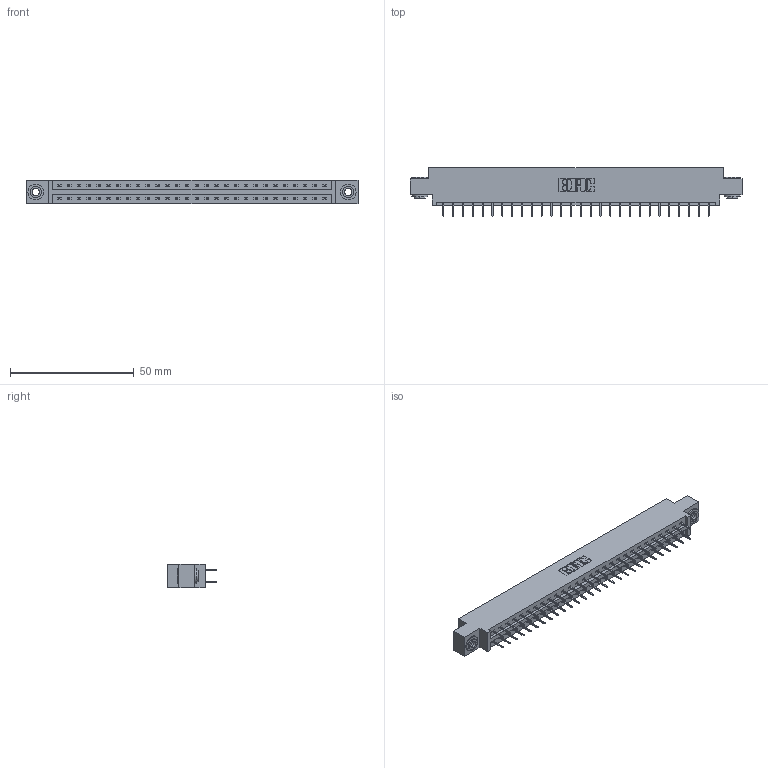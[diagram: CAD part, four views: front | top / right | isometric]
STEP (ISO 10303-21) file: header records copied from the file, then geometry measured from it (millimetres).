
FILE_DESCRIPTION (( 'STEP AP203' ), '1' );
FILE_NAME ('387-056-524-803.STEP', '2019-10-19T06:42:10', ( '' ), ( '' ), 'SwSTEP 2.0', 'SolidWorks 2016', '' );
FILE_SCHEMA (( 'CONFIG_CONTROL_DESIGN' ));
Length unit declared in the file: inch
Products named in the file (4): 337 Part_0.170 Offset - 0.156 Dia-TH; 345-250-002_345-250-002-102; 387-056-524-803; 345-292-001_345-293-124
Assembly tree (59 placements, depth 2):
  387-056-524-803
    337 Part_0.170 Offset - 0.156 Dia-TH
    345-292-001_345-293-124  x56
    345-250-002_345-250-002-102  x2
Bounding box: 133.96 x 19.69 x 9.4 mm (x, y, z)
Volume: 13748.5 mm3; surface area: 15476.5 mm2
Topology: 59 solids, 59 shells, 3404 faces, 9639 edges, 6198 vertices
Faces by surface type: plane 2548, cylinder 848, cone 8
Entity records: 24376 total; most frequent: CARTESIAN_POINT 4093, ORIENTED_EDGE 4022, DIRECTION 3541, EDGE_CURVE 2011, LINE 1863, VECTOR 1863, VERTEX_POINT 1334, AXIS2_PLACEMENT_3D 839
